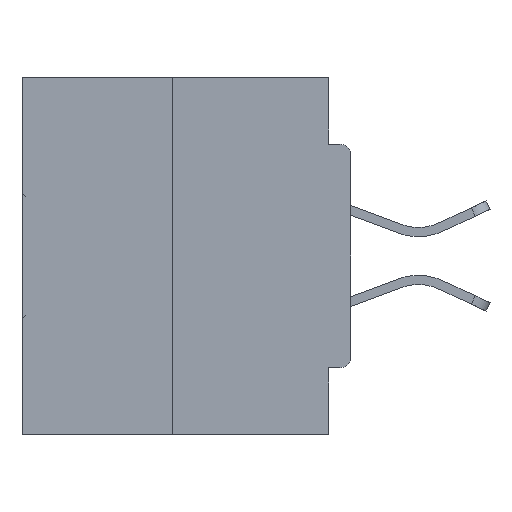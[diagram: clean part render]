
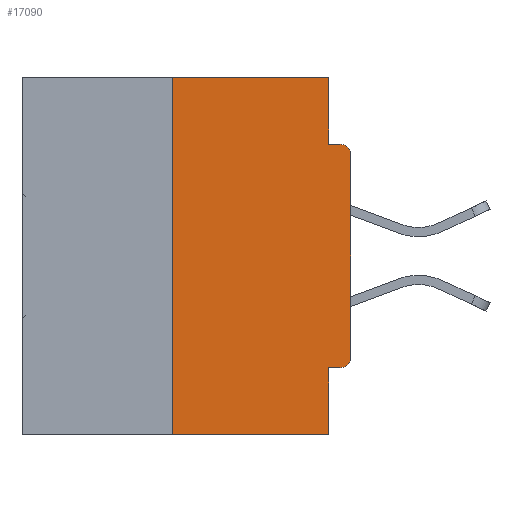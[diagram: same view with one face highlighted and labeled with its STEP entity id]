
A CAD part, left-side view. The second image highlights one B-rep face of the part: STEP entity #17090.
In plain terms, the highlighted planar face has unit normal (-1, 0, 0).
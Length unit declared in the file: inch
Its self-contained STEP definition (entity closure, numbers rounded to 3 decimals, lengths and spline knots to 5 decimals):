
#236 = LINE ( 'NONE', #31582, #10635 ) ;
#1089 = CARTESIAN_POINT ( 'NONE',  ( 0., 0.031, -0.5 ) ) ;
#1497 = DIRECTION ( 'NONE',  ( 0., -1., 0. ) ) ;
#2389 = CARTESIAN_POINT ( 'NONE',  ( 0., 0.031, 0. ) ) ;
#3072 = VECTOR ( 'NONE', #1497, 39.37008 ) ;
#3771 = CARTESIAN_POINT ( 'NONE',  ( 0., 0.031, 0. ) ) ;
#3909 = CARTESIAN_POINT ( 'NONE',  ( 0., 0.25, 0. ) ) ;
#3966 = CARTESIAN_POINT ( 'NONE',  ( 0., 0.031, -0.4065 ) ) ;
#3978 = EDGE_CURVE ( 'NONE', #31526, #4923, #42979, .T. ) ;
#4090 = DIRECTION ( 'NONE',  ( 0., 0., -1. ) ) ;
#4720 = VERTEX_POINT ( 'NONE', #24196 ) ;
#4923 = VERTEX_POINT ( 'NONE', #39990 ) ;
#5381 = ORIENTED_EDGE ( 'NONE', *, *, #22695, .F. ) ;
#5638 = CARTESIAN_POINT ( 'NONE',  ( 0., 0.015, -0.1085 ) ) ;
#6211 = EDGE_CURVE ( 'NONE', #31526, #10860, #24644, .T. ) ;
#8052 = DIRECTION ( 'NONE',  ( 0., 0., -1. ) ) ;
#9548 = EDGE_CURVE ( 'NONE', #24105, #35654, #22828, .T. ) ;
#9989 = ORIENTED_EDGE ( 'NONE', *, *, #6211, .F. ) ;
#10544 = LINE ( 'NONE', #34032, #22008 ) ;
#10635 = VECTOR ( 'NONE', #18518, 39.37008 ) ;
#10860 = VERTEX_POINT ( 'NONE', #3966 ) ;
#11199 = CARTESIAN_POINT ( 'NONE',  ( 0., 0.25, -0.5 ) ) ;
#11550 = PLANE ( 'NONE',  #39537 ) ;
#11688 = CIRCLE ( 'NONE', #32534, 0.015 ) ;
#12471 = DIRECTION ( 'NONE',  ( -1., 0., 0. ) ) ;
#12547 = ORIENTED_EDGE ( 'NONE', *, *, #14801, .F. ) ;
#13036 = EDGE_CURVE ( 'NONE', #28408, #40060, #30308, .T. ) ;
#13183 = VECTOR ( 'NONE', #30246, 39.37008 ) ;
#14001 = CARTESIAN_POINT ( 'NONE',  ( 0., 0., -0.4065 ) ) ;
#14056 = ORIENTED_EDGE ( 'NONE', *, *, #36993, .F. ) ;
#14078 = DIRECTION ( 'NONE',  ( 0., 0., 1. ) ) ;
#14599 = ORIENTED_EDGE ( 'NONE', *, *, #26927, .T. ) ;
#14686 = ORIENTED_EDGE ( 'NONE', *, *, #13036, .F. ) ;
#14801 = EDGE_CURVE ( 'NONE', #10860, #35654, #236, .T. ) ;
#14974 = VECTOR ( 'NONE', #31389, 39.37008 ) ;
#14990 = CARTESIAN_POINT ( 'NONE',  ( 0., 0., -0.0935 ) ) ;
#15005 = VERTEX_POINT ( 'NONE', #2389 ) ;
#16878 = CARTESIAN_POINT ( 'NONE',  ( 0., 0.015, -0.0935 ) ) ;
#16895 = LINE ( 'NONE', #3771, #42927 ) ;
#17090 = ADVANCED_FACE ( 'NONE', ( #25075 ), #11550, .F. ) ;
#17112 = EDGE_LOOP ( 'NONE', ( #5381, #35870, #35193, #12547, #9989, #19813, #29897, #14599, #14686, #14056 ) ) ;
#18518 = DIRECTION ( 'NONE',  ( 0., 0., -1. ) ) ;
#19030 = DIRECTION ( 'NONE',  ( -1., 0., 0. ) ) ;
#19259 = DIRECTION ( 'NONE',  ( 0., 0., -1. ) ) ;
#19813 = ORIENTED_EDGE ( 'NONE', *, *, #3978, .T. ) ;
#20897 = EDGE_CURVE ( 'NONE', #24105, #26172, #31823, .T. ) ;
#22008 = VECTOR ( 'NONE', #34171, 39.37008 ) ;
#22695 = EDGE_CURVE ( 'NONE', #26172, #15005, #31621, .T. ) ;
#22828 = LINE ( 'NONE', #37930, #3072 ) ;
#24105 = VERTEX_POINT ( 'NONE', #11199 ) ;
#24196 = CARTESIAN_POINT ( 'NONE',  ( 0., 0., -0.1085 ) ) ;
#24644 = LINE ( 'NONE', #14001, #13183 ) ;
#25075 = FACE_OUTER_BOUND ( 'NONE', #17112, .T. ) ;
#26172 = VERTEX_POINT ( 'NONE', #39824 ) ;
#26927 = EDGE_CURVE ( 'NONE', #4720, #40060, #11688, .T. ) ;
#27284 = CARTESIAN_POINT ( 'NONE',  ( 0., 0.015, -0.4065 ) ) ;
#28408 = VERTEX_POINT ( 'NONE', #39829 ) ;
#28777 = DIRECTION ( 'NONE',  ( 0., -1., 0. ) ) ;
#29897 = ORIENTED_EDGE ( 'NONE', *, *, #43036, .T. ) ;
#30246 = DIRECTION ( 'NONE',  ( 0., 1., 0. ) ) ;
#30308 = LINE ( 'NONE', #14990, #34476 ) ;
#31389 = DIRECTION ( 'NONE',  ( 0., -1., 0. ) ) ;
#31526 = VERTEX_POINT ( 'NONE', #27284 ) ;
#31582 = CARTESIAN_POINT ( 'NONE',  ( 0., 0.031, -0.5 ) ) ;
#31621 = LINE ( 'NONE', #41308, #14974 ) ;
#31823 = LINE ( 'NONE', #3909, #32310 ) ;
#32310 = VECTOR ( 'NONE', #14078, 39.37008 ) ;
#32534 = AXIS2_PLACEMENT_3D ( 'NONE', #5638, #12471, #19259 ) ;
#34032 = CARTESIAN_POINT ( 'NONE',  ( 0., 0., 0. ) ) ;
#34171 = DIRECTION ( 'NONE',  ( 0., 0., 1. ) ) ;
#34476 = VECTOR ( 'NONE', #28777, 39.37008 ) ;
#34602 = CARTESIAN_POINT ( 'NONE',  ( 0., 0.46, 0. ) ) ;
#35193 = ORIENTED_EDGE ( 'NONE', *, *, #9548, .T. ) ;
#35654 = VERTEX_POINT ( 'NONE', #1089 ) ;
#35870 = ORIENTED_EDGE ( 'NONE', *, *, #20897, .F. ) ;
#36993 = EDGE_CURVE ( 'NONE', #15005, #28408, #16895, .T. ) ;
#37761 = AXIS2_PLACEMENT_3D ( 'NONE', #38955, #19030, #42311 ) ;
#37827 = DIRECTION ( 'NONE',  ( 1., 0., 0. ) ) ;
#37930 = CARTESIAN_POINT ( 'NONE',  ( 0., 0.46, -0.5 ) ) ;
#38955 = CARTESIAN_POINT ( 'NONE',  ( 0., 0.015, -0.3915 ) ) ;
#39537 = AXIS2_PLACEMENT_3D ( 'NONE', #34602, #37827, #8052 ) ;
#39824 = CARTESIAN_POINT ( 'NONE',  ( 0., 0.25, 0. ) ) ;
#39829 = CARTESIAN_POINT ( 'NONE',  ( 0., 0.031, -0.0935 ) ) ;
#39990 = CARTESIAN_POINT ( 'NONE',  ( 0., 0., -0.3915 ) ) ;
#40060 = VERTEX_POINT ( 'NONE', #16878 ) ;
#41308 = CARTESIAN_POINT ( 'NONE',  ( 0., 0.46, 0. ) ) ;
#42311 = DIRECTION ( 'NONE',  ( 0., 0., -1. ) ) ;
#42927 = VECTOR ( 'NONE', #4090, 39.37008 ) ;
#42979 = CIRCLE ( 'NONE', #37761, 0.015 ) ;
#43036 = EDGE_CURVE ( 'NONE', #4923, #4720, #10544, .T. ) ;
